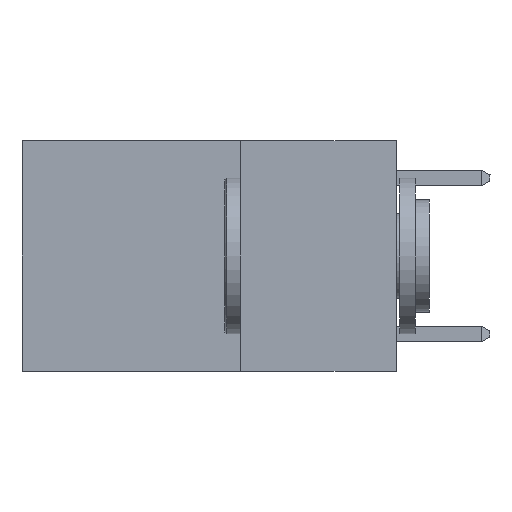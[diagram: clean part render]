
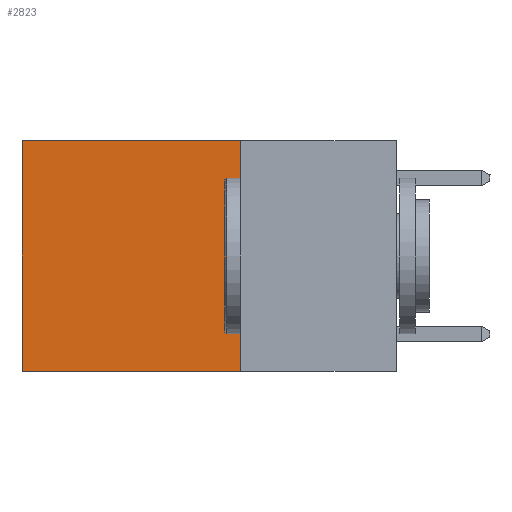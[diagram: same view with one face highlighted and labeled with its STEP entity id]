
A CAD part, left-side view. The second image highlights one B-rep face of the part: STEP entity #2823.
In plain terms, the highlighted planar face has unit normal (-1, 0, 0).
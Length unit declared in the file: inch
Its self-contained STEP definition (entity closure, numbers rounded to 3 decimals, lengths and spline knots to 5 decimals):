
#148 = EDGE_CURVE ( 'NONE', #6040, #3616, #5609, .T. ) ;
#210 = EDGE_CURVE ( 'NONE', #3616, #1868, #6722, .T. ) ;
#459 = VECTOR ( 'NONE', #1530, 39.37008 ) ;
#600 = EDGE_CURVE ( 'NONE', #5662, #1868, #7135, .T. ) ;
#620 = CARTESIAN_POINT ( 'NONE',  ( 0.2625, 0.25, -0.37 ) ) ;
#1530 = DIRECTION ( 'NONE',  ( 0., 1., 0. ) ) ;
#1852 = CARTESIAN_POINT ( 'NONE',  ( 0.2625, 0.25, -0.37 ) ) ;
#1868 = VERTEX_POINT ( 'NONE', #2675 ) ;
#2012 = CARTESIAN_POINT ( 'NONE',  ( 0.2625, 0.6, 0. ) ) ;
#2381 = ORIENTED_EDGE ( 'NONE', *, *, #600, .T. ) ;
#2510 = EDGE_CURVE ( 'NONE', #6040, #5662, #7032, .T. ) ;
#2530 = EDGE_LOOP ( 'NONE', ( #2381, #4557, #9090, #3220 ) ) ;
#2675 = CARTESIAN_POINT ( 'NONE',  ( 0.2625, 0.6, -0.37 ) ) ;
#2823 = ADVANCED_FACE ( 'NONE', ( #9427 ), #8564, .F. ) ;
#3220 = ORIENTED_EDGE ( 'NONE', *, *, #2510, .T. ) ;
#3537 = DIRECTION ( 'NONE',  ( 1., 0., 0. ) ) ;
#3616 = VERTEX_POINT ( 'NONE', #1852 ) ;
#3752 = DIRECTION ( 'NONE',  ( 0., 0., -1. ) ) ;
#4421 = CARTESIAN_POINT ( 'NONE',  ( 0.2625, 0.25, 0. ) ) ;
#4557 = ORIENTED_EDGE ( 'NONE', *, *, #210, .F. ) ;
#4602 = DIRECTION ( 'NONE',  ( 0., 0., -1. ) ) ;
#5069 = VECTOR ( 'NONE', #8703, 39.37008 ) ;
#5609 = LINE ( 'NONE', #7211, #7668 ) ;
#5662 = VERTEX_POINT ( 'NONE', #8977 ) ;
#6011 = CARTESIAN_POINT ( 'NONE',  ( 0.2625, 0.25, 0. ) ) ;
#6040 = VERTEX_POINT ( 'NONE', #8835 ) ;
#6722 = LINE ( 'NONE', #620, #459 ) ;
#6969 = VECTOR ( 'NONE', #7675, 39.37008 ) ;
#7032 = LINE ( 'NONE', #6011, #6969 ) ;
#7089 = AXIS2_PLACEMENT_3D ( 'NONE', #4421, #3537, #4602 ) ;
#7135 = LINE ( 'NONE', #2012, #5069 ) ;
#7211 = CARTESIAN_POINT ( 'NONE',  ( 0.2625, 0.25, 0. ) ) ;
#7668 = VECTOR ( 'NONE', #3752, 39.37008 ) ;
#7675 = DIRECTION ( 'NONE',  ( 0., 1., 0. ) ) ;
#8564 = PLANE ( 'NONE',  #7089 ) ;
#8703 = DIRECTION ( 'NONE',  ( 0., 0., -1. ) ) ;
#8835 = CARTESIAN_POINT ( 'NONE',  ( 0.2625, 0.25, 0. ) ) ;
#8977 = CARTESIAN_POINT ( 'NONE',  ( 0.2625, 0.6, 0. ) ) ;
#9090 = ORIENTED_EDGE ( 'NONE', *, *, #148, .F. ) ;
#9427 = FACE_OUTER_BOUND ( 'NONE', #2530, .T. ) ;
